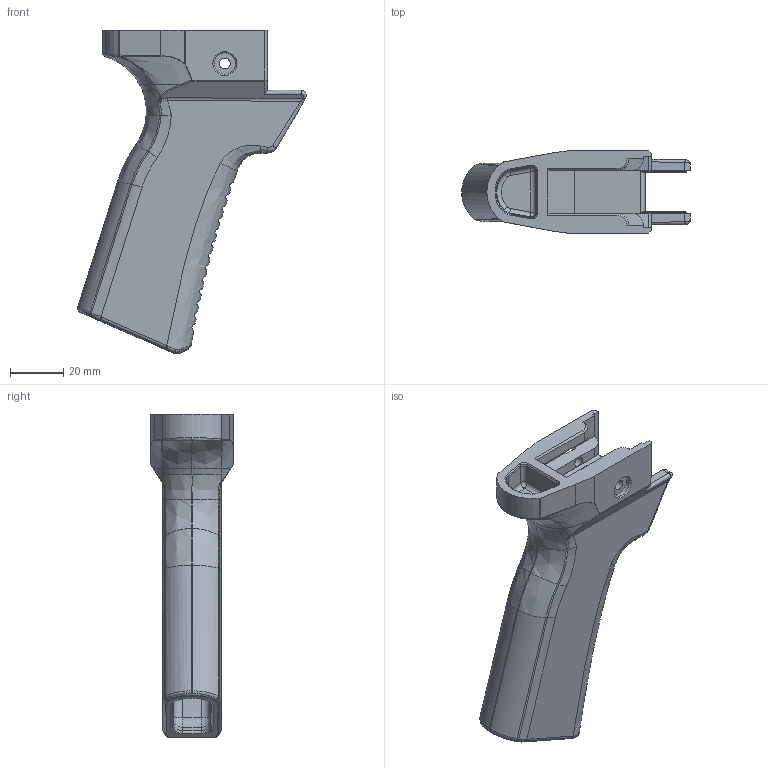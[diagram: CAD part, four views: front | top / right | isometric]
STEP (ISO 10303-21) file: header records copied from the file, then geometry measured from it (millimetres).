
FILE_DESCRIPTION(/* description */ (''),/* implementation_level */ '2;1');
FILE_NAME(/* name */ 'Evo Contoured Grip.step',/* time_stamp */ '2021-08-29T20:14:05-04:00',/* author */ (''),/* organization */ (''),/* preprocessor_version */ 'ST-DEVELOPER v18.1',/* originating_system */ 'Autodesk Translation Framework v10.10.0.1391',/* authorisation */ '');
FILE_SCHEMA (('AUTOMOTIVE_DESIGN { 1 0 10303 214 3 1 1 }'));
Length unit declared in the file: millimetre
Products named in the file (1): Thin Contour Grip
Bounding box: 85.91 x 31 x 121.67 mm (x, y, z)
Volume: 65236.8 mm3; surface area: 28733.1 mm2
Topology: 1 solids, 1 shells, 499 faces, 1265 edges, 757 vertices
Faces by surface type: bspline 198, cylinder 126, plane 107, torus 42, sphere 16, cone 10
Full cylindrical faces by diameter (mm): 4 x2, 8 x1
Entity records: 25908 total; most frequent: CARTESIAN_POINT 15323, ORIENTED_EDGE 2502, DIRECTION 1717, EDGE_CURVE 1251, VERTEX_POINT 757, AXIS2_PLACEMENT_3D 654, EDGE_LOOP 510, FACE_OUTER_BOUND 499
